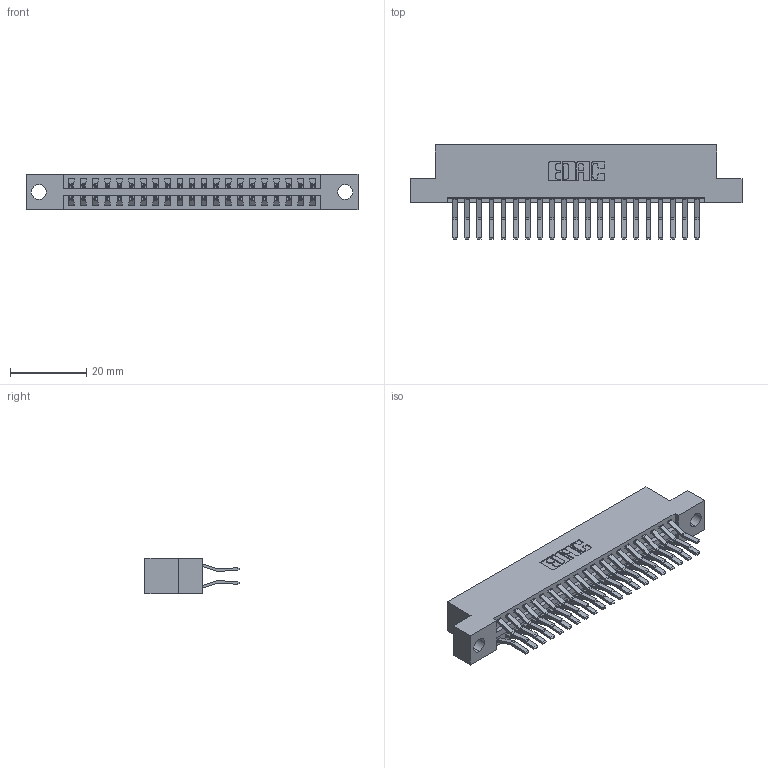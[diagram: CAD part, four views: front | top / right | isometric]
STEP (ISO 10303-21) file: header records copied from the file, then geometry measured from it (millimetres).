
FILE_DESCRIPTION (( 'STEP AP203' ), '1' );
FILE_NAME ('396-042-560-204.STEP', '2018-09-07T01:41:18', ( '' ), ( '' ), 'SwSTEP 2.0', 'SolidWorks 2016', '' );
FILE_SCHEMA (( 'CONFIG_CONTROL_DESIGN' ));
Length unit declared in the file: inch
Products named in the file (3): 396-042-560-204; 346 Part_Flush Mounting Lugs - 0.156 Dia-TH; 345-292-001_560 Tail
Assembly tree (43 placements, depth 2):
  396-042-560-204
    346 Part_Flush Mounting Lugs - 0.156 Dia-TH
    345-292-001_560 Tail  x42
Bounding box: 87.25 x 24.78 x 9.4 mm (x, y, z)
Volume: 8532.2 mm3; surface area: 11945.8 mm2
Topology: 43 solids, 43 shells, 2390 faces, 7091 edges, 4670 vertices
Faces by surface type: plane 1546, cylinder 844
Entity records: 16623 total; most frequent: CARTESIAN_POINT 2768, ORIENTED_EDGE 2702, DIRECTION 2495, EDGE_CURVE 1351, LINE 1131, VECTOR 1131, VERTEX_POINT 898, AXIS2_PLACEMENT_3D 682
